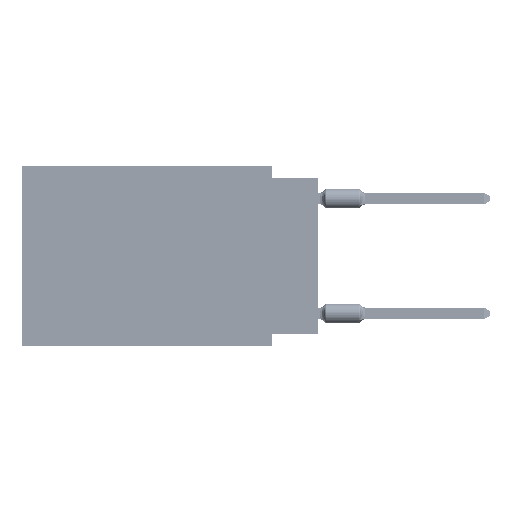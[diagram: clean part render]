
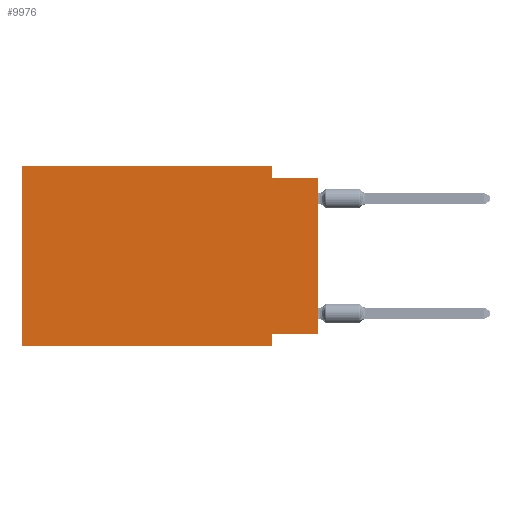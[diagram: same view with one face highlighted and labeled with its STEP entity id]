
A CAD part, left-side view. The second image highlights one B-rep face of the part: STEP entity #9976.
In plain terms, the highlighted planar face has unit normal (-1, 0, 0).
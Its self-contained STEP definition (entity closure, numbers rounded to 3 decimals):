
#3275 = DIRECTION ( 'NONE',  ( 0., 0., -1. ) ) ;
#3442 = ORIENTED_EDGE ( 'NONE', *, *, #51192, .F. ) ;
#6619 = DIRECTION ( 'NONE',  ( 0., 0., 1. ) ) ;
#6918 = VECTOR ( 'NONE', #53354, 1000. ) ;
#8030 = DIRECTION ( 'NONE',  ( 0., 0., -1. ) ) ;
#8490 = VECTOR ( 'NONE', #10289, 1000. ) ;
#8952 = EDGE_CURVE ( 'NONE', #56388, #50438, #10654, .T. ) ;
#9976 = ADVANCED_FACE ( 'NONE', ( #14387 ), #55116, .F. ) ;
#10289 = DIRECTION ( 'NONE',  ( 0., -1., 0. ) ) ;
#10654 = LINE ( 'NONE', #66965, #8490 ) ;
#13098 = ORIENTED_EDGE ( 'NONE', *, *, #8952, .F. ) ;
#14184 = CARTESIAN_POINT ( 'NONE',  ( 0., 2.54, -9.906 ) ) ;
#14387 = FACE_OUTER_BOUND ( 'NONE', #51913, .T. ) ;
#16125 = VERTEX_POINT ( 'NONE', #29868 ) ;
#17436 = CARTESIAN_POINT ( 'NONE',  ( 0., 16.383, 0. ) ) ;
#17536 = VECTOR ( 'NONE', #6619, 1000. ) ;
#17845 = VERTEX_POINT ( 'NONE', #17436 ) ;
#19088 = ORIENTED_EDGE ( 'NONE', *, *, #42464, .T. ) ;
#19683 = VERTEX_POINT ( 'NONE', #54340 ) ;
#19759 = VECTOR ( 'NONE', #56049, 1000. ) ;
#20342 = LINE ( 'NONE', #58867, #35093 ) ;
#22515 = CARTESIAN_POINT ( 'NONE',  ( 0., 2.54, -9.271 ) ) ;
#24728 = CARTESIAN_POINT ( 'NONE',  ( 0., 16.383, 0. ) ) ;
#24960 = DIRECTION ( 'NONE',  ( 0., 0., -1. ) ) ;
#25506 = DIRECTION ( 'NONE',  ( 1., 0., 0. ) ) ;
#27680 = LINE ( 'NONE', #14184, #31213 ) ;
#28413 = VERTEX_POINT ( 'NONE', #64451 ) ;
#28804 = LINE ( 'NONE', #31709, #33483 ) ;
#29258 = CARTESIAN_POINT ( 'NONE',  ( 0., 0., -0.635 ) ) ;
#29553 = DIRECTION ( 'NONE',  ( 0., -1., 0. ) ) ;
#29868 = CARTESIAN_POINT ( 'NONE',  ( 0., 16.383, -9.906 ) ) ;
#31213 = VECTOR ( 'NONE', #24960, 1000. ) ;
#31709 = CARTESIAN_POINT ( 'NONE',  ( 0., 2.54, 0. ) ) ;
#33459 = CARTESIAN_POINT ( 'NONE',  ( 0., 0., -9.271 ) ) ;
#33483 = VECTOR ( 'NONE', #8030, 1000. ) ;
#33557 = EDGE_CURVE ( 'NONE', #17845, #28413, #63282, .T. ) ;
#33559 = CARTESIAN_POINT ( 'NONE',  ( 0., 2.54, -0.635 ) ) ;
#35093 = VECTOR ( 'NONE', #47748, 1000. ) ;
#35752 = AXIS2_PLACEMENT_3D ( 'NONE', #60693, #25506, #3275 ) ;
#36800 = EDGE_CURVE ( 'NONE', #28413, #56388, #28804, .T. ) ;
#37610 = ORIENTED_EDGE ( 'NONE', *, *, #52462, .F. ) ;
#42464 = EDGE_CURVE ( 'NONE', #16125, #68880, #20342, .T. ) ;
#47748 = DIRECTION ( 'NONE',  ( 0., -1., 0. ) ) ;
#49231 = ORIENTED_EDGE ( 'NONE', *, *, #36800, .F. ) ;
#50438 = VERTEX_POINT ( 'NONE', #29258 ) ;
#50699 = LINE ( 'NONE', #67769, #17536 ) ;
#51192 = EDGE_CURVE ( 'NONE', #19683, #64792, #73097, .T. ) ;
#51913 = EDGE_LOOP ( 'NONE', ( #70465, #13098, #49231, #54910, #37610, #19088, #57157, #3442 ) ) ;
#52462 = EDGE_CURVE ( 'NONE', #16125, #17845, #70402, .T. ) ;
#52472 = CARTESIAN_POINT ( 'NONE',  ( 0., 2.54, -9.906 ) ) ;
#52672 = EDGE_CURVE ( 'NONE', #19683, #50438, #50699, .T. ) ;
#53354 = DIRECTION ( 'NONE',  ( 0., 0., 1. ) ) ;
#54340 = CARTESIAN_POINT ( 'NONE',  ( 0., 0., -9.271 ) ) ;
#54910 = ORIENTED_EDGE ( 'NONE', *, *, #33557, .F. ) ;
#55116 = PLANE ( 'NONE',  #35752 ) ;
#56049 = DIRECTION ( 'NONE',  ( 0., 1., 0. ) ) ;
#56388 = VERTEX_POINT ( 'NONE', #33559 ) ;
#57157 = ORIENTED_EDGE ( 'NONE', *, *, #72855, .F. ) ;
#58867 = CARTESIAN_POINT ( 'NONE',  ( 0., 16.383, -9.906 ) ) ;
#60693 = CARTESIAN_POINT ( 'NONE',  ( 0., 16.383, 0. ) ) ;
#63282 = LINE ( 'NONE', #24728, #71230 ) ;
#64451 = CARTESIAN_POINT ( 'NONE',  ( 0., 2.54, 0. ) ) ;
#64792 = VERTEX_POINT ( 'NONE', #22515 ) ;
#64842 = CARTESIAN_POINT ( 'NONE',  ( 0., 16.383, 0. ) ) ;
#66965 = CARTESIAN_POINT ( 'NONE',  ( 0., 0., -0.635 ) ) ;
#67769 = CARTESIAN_POINT ( 'NONE',  ( 0., 0., 0. ) ) ;
#68880 = VERTEX_POINT ( 'NONE', #52472 ) ;
#70402 = LINE ( 'NONE', #64842, #6918 ) ;
#70465 = ORIENTED_EDGE ( 'NONE', *, *, #52672, .T. ) ;
#71230 = VECTOR ( 'NONE', #29553, 1000. ) ;
#72855 = EDGE_CURVE ( 'NONE', #64792, #68880, #27680, .T. ) ;
#73097 = LINE ( 'NONE', #33459, #19759 ) ;
